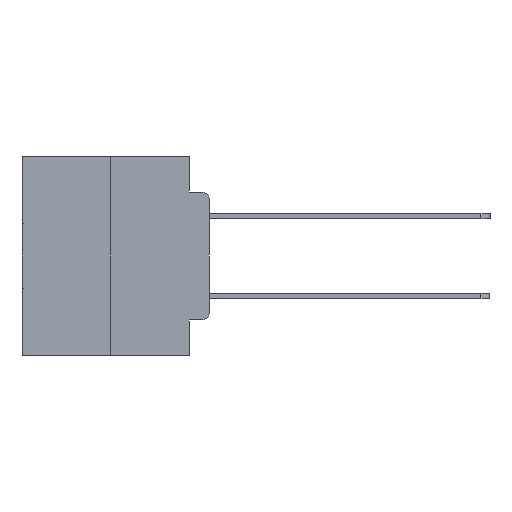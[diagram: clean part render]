
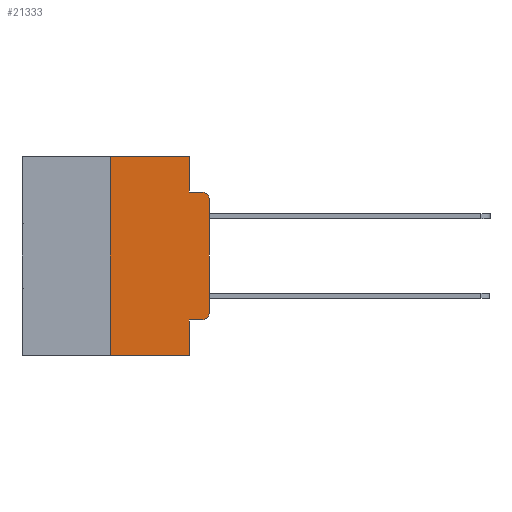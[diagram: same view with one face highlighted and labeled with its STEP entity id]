
A CAD part, left-side view. The second image highlights one B-rep face of the part: STEP entity #21333.
In plain terms, the highlighted planar face has unit normal (-1, 0, 0).
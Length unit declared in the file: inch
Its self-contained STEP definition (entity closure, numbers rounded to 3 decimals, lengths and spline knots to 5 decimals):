
#224 = VERTEX_POINT ( 'NONE', #11277 ) ;
#701 = ORIENTED_EDGE ( 'NONE', *, *, #5230, .T. ) ;
#1102 = DIRECTION ( 'NONE',  ( 0., -1., 0. ) ) ;
#1987 = DIRECTION ( 'NONE',  ( -1., 0., 0. ) ) ;
#2026 = CIRCLE ( 'NONE', #20343, 0.02 ) ;
#2119 = EDGE_CURVE ( 'NONE', #27997, #19373, #12666, .T. ) ;
#2599 = CARTESIAN_POINT ( 'NONE',  ( 0., 0., -0.1085 ) ) ;
#2825 = DIRECTION ( 'NONE',  ( 1., 0., 0. ) ) ;
#2969 = EDGE_LOOP ( 'NONE', ( #701, #18667, #27829, #19925, #3984, #23367, #19391, #16063, #4699, #23120 ) ) ;
#3580 = CARTESIAN_POINT ( 'NONE',  ( 0., 0., -0.3915 ) ) ;
#3843 = CARTESIAN_POINT ( 'NONE',  ( 0., 0.02, -0.1085 ) ) ;
#3984 = ORIENTED_EDGE ( 'NONE', *, *, #11531, .F. ) ;
#4496 = DIRECTION ( 'NONE',  ( 0., -1., 0. ) ) ;
#4675 = VERTEX_POINT ( 'NONE', #3580 ) ;
#4699 = ORIENTED_EDGE ( 'NONE', *, *, #20947, .T. ) ;
#4932 = CARTESIAN_POINT ( 'NONE',  ( 0., 0.051, -0.5 ) ) ;
#5230 = EDGE_CURVE ( 'NONE', #4675, #16531, #23666, .T. ) ;
#5294 = DIRECTION ( 'NONE',  ( 0., 0., 1. ) ) ;
#5727 = DIRECTION ( 'NONE',  ( 0., 0., 1. ) ) ;
#6143 = DIRECTION ( 'NONE',  ( 0., 0., -1. ) ) ;
#6456 = VECTOR ( 'NONE', #1102, 39.37008 ) ;
#7053 = CARTESIAN_POINT ( 'NONE',  ( 0., 0.051, -0.0885 ) ) ;
#7156 = VECTOR ( 'NONE', #5294, 39.37008 ) ;
#7693 = VERTEX_POINT ( 'NONE', #18912 ) ;
#8080 = VECTOR ( 'NONE', #21226, 39.37008 ) ;
#8880 = CARTESIAN_POINT ( 'NONE',  ( 0., 0.051, 0. ) ) ;
#9458 = AXIS2_PLACEMENT_3D ( 'NONE', #15651, #1987, #17931 ) ;
#9753 = LINE ( 'NONE', #28061, #26845 ) ;
#11109 = CIRCLE ( 'NONE', #9458, 0.02 ) ;
#11277 = CARTESIAN_POINT ( 'NONE',  ( 0., 0.02, -0.4115 ) ) ;
#11531 = EDGE_CURVE ( 'NONE', #22133, #19480, #20148, .T. ) ;
#11850 = CARTESIAN_POINT ( 'NONE',  ( 0., 0.051, -0.4115 ) ) ;
#11941 = PLANE ( 'NONE',  #19669 ) ;
#12075 = LINE ( 'NONE', #11850, #23267 ) ;
#12177 = LINE ( 'NONE', #21903, #23369 ) ;
#12666 = LINE ( 'NONE', #7053, #23842 ) ;
#12669 = CARTESIAN_POINT ( 'NONE',  ( 0., 0.25, -0.5 ) ) ;
#13445 = FACE_OUTER_BOUND ( 'NONE', #2969, .T. ) ;
#14098 = DIRECTION ( 'NONE',  ( 0., -1., 0. ) ) ;
#14331 = CARTESIAN_POINT ( 'NONE',  ( 0., 0., 0. ) ) ;
#14451 = CARTESIAN_POINT ( 'NONE',  ( 0., 0.051, 0. ) ) ;
#15277 = CARTESIAN_POINT ( 'NONE',  ( 0., 0.02, -0.0885 ) ) ;
#15651 = CARTESIAN_POINT ( 'NONE',  ( 0., 0.02, -0.3915 ) ) ;
#16063 = ORIENTED_EDGE ( 'NONE', *, *, #23899, .F. ) ;
#16245 = DIRECTION ( 'NONE',  ( 0., -1., 0. ) ) ;
#16531 = VERTEX_POINT ( 'NONE', #2599 ) ;
#17090 = CARTESIAN_POINT ( 'NONE',  ( 0., 0.473, -0.5 ) ) ;
#17312 = CARTESIAN_POINT ( 'NONE',  ( 0., 0.25, 0. ) ) ;
#17931 = DIRECTION ( 'NONE',  ( 0., 0., -1. ) ) ;
#18520 = LINE ( 'NONE', #17090, #6456 ) ;
#18667 = ORIENTED_EDGE ( 'NONE', *, *, #27769, .T. ) ;
#18693 = EDGE_CURVE ( 'NONE', #26083, #19643, #18520, .T. ) ;
#18734 = DIRECTION ( 'NONE',  ( 0., 0., -1. ) ) ;
#18776 = VECTOR ( 'NONE', #16245, 39.37008 ) ;
#18912 = CARTESIAN_POINT ( 'NONE',  ( 0., 0.051, -0.4115 ) ) ;
#19373 = VERTEX_POINT ( 'NONE', #15277 ) ;
#19391 = ORIENTED_EDGE ( 'NONE', *, *, #18693, .T. ) ;
#19465 = EDGE_CURVE ( 'NONE', #224, #4675, #11109, .T. ) ;
#19480 = VERTEX_POINT ( 'NONE', #8880 ) ;
#19643 = VERTEX_POINT ( 'NONE', #4932 ) ;
#19669 = AXIS2_PLACEMENT_3D ( 'NONE', #27505, #2825, #18734 ) ;
#19701 = DIRECTION ( 'NONE',  ( -1., 0., 0. ) ) ;
#19925 = ORIENTED_EDGE ( 'NONE', *, *, #28325, .F. ) ;
#20148 = LINE ( 'NONE', #27294, #18776 ) ;
#20343 = AXIS2_PLACEMENT_3D ( 'NONE', #3843, #19701, #6143 ) ;
#20947 = EDGE_CURVE ( 'NONE', #7693, #224, #12075, .T. ) ;
#21226 = DIRECTION ( 'NONE',  ( 0., 0., -1. ) ) ;
#21333 = ADVANCED_FACE ( 'NONE', ( #13445 ), #11941, .F. ) ;
#21903 = CARTESIAN_POINT ( 'NONE',  ( 0., 0.051, 0. ) ) ;
#22133 = VERTEX_POINT ( 'NONE', #17312 ) ;
#23120 = ORIENTED_EDGE ( 'NONE', *, *, #19465, .T. ) ;
#23267 = VECTOR ( 'NONE', #14098, 39.37008 ) ;
#23367 = ORIENTED_EDGE ( 'NONE', *, *, #25373, .F. ) ;
#23369 = VECTOR ( 'NONE', #24123, 39.37008 ) ;
#23666 = LINE ( 'NONE', #14331, #7156 ) ;
#23842 = VECTOR ( 'NONE', #4496, 39.37008 ) ;
#23899 = EDGE_CURVE ( 'NONE', #7693, #19643, #25920, .T. ) ;
#24123 = DIRECTION ( 'NONE',  ( 0., 0., -1. ) ) ;
#25373 = EDGE_CURVE ( 'NONE', #26083, #22133, #9753, .T. ) ;
#25920 = LINE ( 'NONE', #14451, #8080 ) ;
#26083 = VERTEX_POINT ( 'NONE', #12669 ) ;
#26845 = VECTOR ( 'NONE', #5727, 39.37008 ) ;
#27004 = CARTESIAN_POINT ( 'NONE',  ( 0., 0.051, -0.0885 ) ) ;
#27294 = CARTESIAN_POINT ( 'NONE',  ( 0., 0.473, 0. ) ) ;
#27505 = CARTESIAN_POINT ( 'NONE',  ( 0., 0.473, 0. ) ) ;
#27769 = EDGE_CURVE ( 'NONE', #16531, #19373, #2026, .T. ) ;
#27829 = ORIENTED_EDGE ( 'NONE', *, *, #2119, .F. ) ;
#27997 = VERTEX_POINT ( 'NONE', #27004 ) ;
#28061 = CARTESIAN_POINT ( 'NONE',  ( 0., 0.25, 0. ) ) ;
#28325 = EDGE_CURVE ( 'NONE', #19480, #27997, #12177, .T. ) ;
